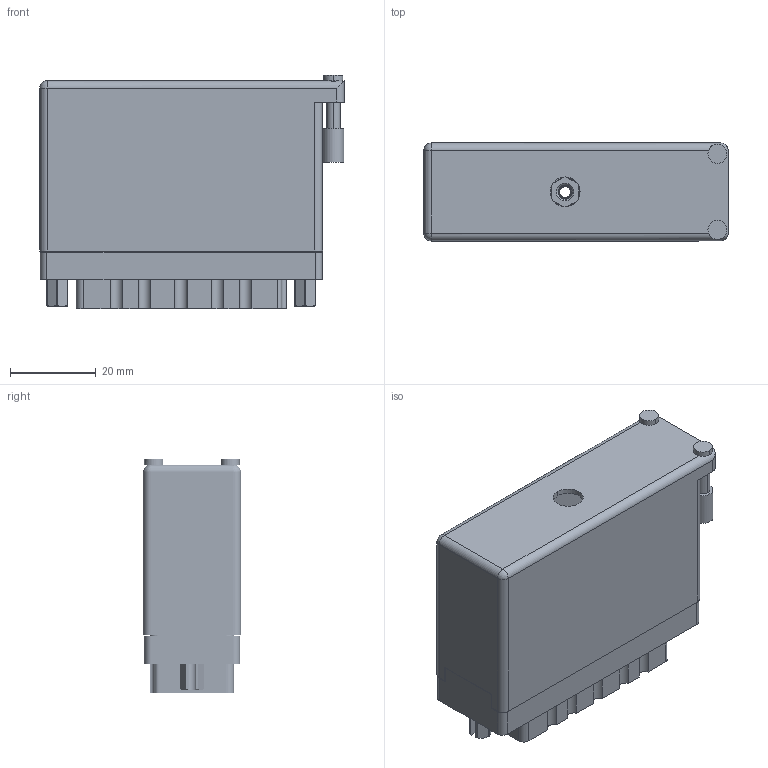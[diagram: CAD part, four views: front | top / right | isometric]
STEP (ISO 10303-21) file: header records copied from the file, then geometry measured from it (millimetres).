
FILE_DESCRIPTION (( 'STEP AP203' ), '1' );
FILE_NAME ('516-056-520-252.STEP', '2020-03-05T23:28:14', ( '' ), ( '' ), 'SwSTEP 2.0', 'SolidWorks 2016', '' );
FILE_SCHEMA (( 'CONFIG_CONTROL_DESIGN' ));
Length unit declared in the file: inch
Products named in the file (8): 516-292-001_520 Contact; 516-221-038-102_056; 516-252-021-102_056; 516-230-001_Metal - 056 Side Entry; 516-221-038-102_057; 516 Part Receptacle_056; 516-056-520-252; 516-252-035-100_516-252-035-100
Assembly tree (63 placements, depth 2):
  516-056-520-252
    516 Part Receptacle_056
    516-292-001_520 Contact  x56
    516-230-001_Metal - 056 Side Entry
    516-252-021-102_056  x2
    516-221-038-102_056
    516-252-035-100_516-252-035-100
    516-221-038-102_057
Bounding box: 71.12 x 22.83 x 54.53 mm (x, y, z)
Volume: 27181.8 mm3; surface area: 46905.1 mm2
Topology: 63 solids, 63 shells, 5580 faces, 16147 edges, 10708 vertices
Faces by surface type: plane 3336, cylinder 1828, bspline 370, cone 44, sphere 2
Entity records: 61884 total; most frequent: CARTESIAN_POINT 16646, ORIENTED_EDGE 9222, DIRECTION 8789, EDGE_CURVE 4611, VECTOR 3169, LINE 3169, VERTEX_POINT 3058, AXIS2_PLACEMENT_3D 2810
